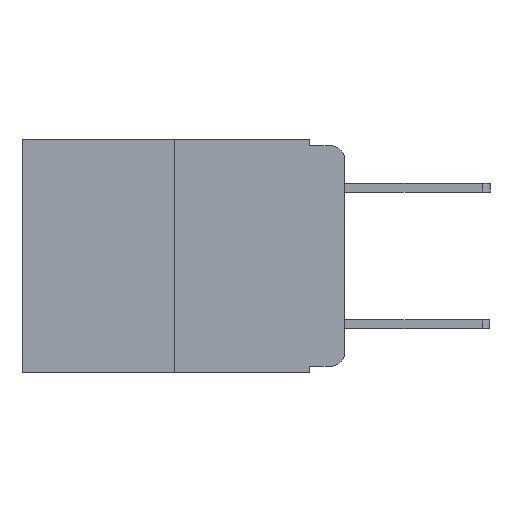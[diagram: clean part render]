
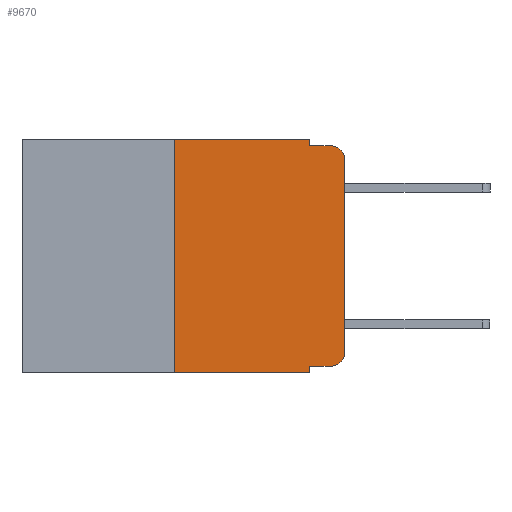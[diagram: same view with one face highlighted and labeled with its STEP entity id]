
A CAD part, left-side view. The second image highlights one B-rep face of the part: STEP entity #9670.
In plain terms, the highlighted planar face has unit normal (-1, 0, 0).
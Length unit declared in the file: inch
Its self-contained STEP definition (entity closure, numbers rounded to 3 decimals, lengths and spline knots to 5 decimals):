
#8 = LINE ( 'NONE', #18733, #17541 ) ;
#516 = DIRECTION ( 'NONE',  ( -1., 0., 0. ) ) ;
#666 = EDGE_CURVE ( 'NONE', #3687, #9447, #8, .T. ) ;
#792 = CARTESIAN_POINT ( 'NONE',  ( 0., 0.051, 0. ) ) ;
#981 = ORIENTED_EDGE ( 'NONE', *, *, #666, .T. ) ;
#1215 = ORIENTED_EDGE ( 'NONE', *, *, #8685, .F. ) ;
#2096 = VERTEX_POINT ( 'NONE', #7950 ) ;
#2182 = CARTESIAN_POINT ( 'NONE',  ( 0., 0.25, 0. ) ) ;
#2945 = EDGE_LOOP ( 'NONE', ( #5885, #19384, #20901, #8991, #1215, #12058, #11297, #17160, #981, #9784 ) ) ;
#3026 = LINE ( 'NONE', #5158, #6870 ) ;
#3411 = VERTEX_POINT ( 'NONE', #9431 ) ;
#3503 = LINE ( 'NONE', #6610, #16013 ) ;
#3687 = VERTEX_POINT ( 'NONE', #15047 ) ;
#3809 = CARTESIAN_POINT ( 'NONE',  ( 0., 0., 0. ) ) ;
#3881 = DIRECTION ( 'NONE',  ( 0., 0., 1. ) ) ;
#3888 = LINE ( 'NONE', #5105, #7714 ) ;
#3938 = VECTOR ( 'NONE', #11403, 39.37008 ) ;
#4030 = LINE ( 'NONE', #3809, #20818 ) ;
#4268 = EDGE_CURVE ( 'NONE', #18880, #7314, #3026, .T. ) ;
#4490 = DIRECTION ( 'NONE',  ( 1., 0., 0. ) ) ;
#4887 = CARTESIAN_POINT ( 'NONE',  ( 0., 0.25, 0. ) ) ;
#5105 = CARTESIAN_POINT ( 'NONE',  ( 0., 0.473, -0.343 ) ) ;
#5158 = CARTESIAN_POINT ( 'NONE',  ( 0., 0.051, 0. ) ) ;
#5649 = DIRECTION ( 'NONE',  ( -1., 0., 0. ) ) ;
#5885 = ORIENTED_EDGE ( 'NONE', *, *, #7518, .T. ) ;
#6610 = CARTESIAN_POINT ( 'NONE',  ( 0., 0.473, 0. ) ) ;
#6811 = DIRECTION ( 'NONE',  ( 0., 0., -1. ) ) ;
#6870 = VECTOR ( 'NONE', #6811, 39.37008 ) ;
#6994 = CIRCLE ( 'NONE', #13100, 0.02 ) ;
#7314 = VERTEX_POINT ( 'NONE', #18001 ) ;
#7518 = EDGE_CURVE ( 'NONE', #12707, #2096, #4030, .T. ) ;
#7714 = VECTOR ( 'NONE', #10047, 39.37008 ) ;
#7950 = CARTESIAN_POINT ( 'NONE',  ( 0., 0., -0.03 ) ) ;
#8685 = EDGE_CURVE ( 'NONE', #11737, #18880, #3503, .T. ) ;
#8953 = VECTOR ( 'NONE', #20118, 39.37008 ) ;
#8991 = ORIENTED_EDGE ( 'NONE', *, *, #4268, .F. ) ;
#9375 = CARTESIAN_POINT ( 'NONE',  ( 0., 0.473, 0. ) ) ;
#9431 = CARTESIAN_POINT ( 'NONE',  ( 0., 0.25, -0.343 ) ) ;
#9438 = LINE ( 'NONE', #792, #20835 ) ;
#9447 = VERTEX_POINT ( 'NONE', #15290 ) ;
#9456 = CARTESIAN_POINT ( 'NONE',  ( 0., 0.02, -0.01 ) ) ;
#9472 = LINE ( 'NONE', #18502, #8953 ) ;
#9670 = ADVANCED_FACE ( 'NONE', ( #18740 ), #20707, .F. ) ;
#9784 = ORIENTED_EDGE ( 'NONE', *, *, #10761, .T. ) ;
#10047 = DIRECTION ( 'NONE',  ( 0., -1., 0. ) ) ;
#10443 = CARTESIAN_POINT ( 'NONE',  ( 0., 0.02, -0.03 ) ) ;
#10444 = EDGE_CURVE ( 'NONE', #3411, #11737, #16956, .T. ) ;
#10761 = EDGE_CURVE ( 'NONE', #9447, #12707, #6994, .T. ) ;
#11297 = ORIENTED_EDGE ( 'NONE', *, *, #21209, .T. ) ;
#11338 = EDGE_CURVE ( 'NONE', #2096, #17224, #17426, .T. ) ;
#11403 = DIRECTION ( 'NONE',  ( 0., 0., 1. ) ) ;
#11737 = VERTEX_POINT ( 'NONE', #2182 ) ;
#12058 = ORIENTED_EDGE ( 'NONE', *, *, #10444, .F. ) ;
#12079 = DIRECTION ( 'NONE',  ( 0., 0., -1. ) ) ;
#12707 = VERTEX_POINT ( 'NONE', #18022 ) ;
#12909 = EDGE_CURVE ( 'NONE', #7314, #17224, #9472, .T. ) ;
#13100 = AXIS2_PLACEMENT_3D ( 'NONE', #15450, #5649, #17083 ) ;
#13389 = AXIS2_PLACEMENT_3D ( 'NONE', #10443, #516, #12079 ) ;
#14003 = CARTESIAN_POINT ( 'NONE',  ( 0., 0.051, -0.343 ) ) ;
#15047 = CARTESIAN_POINT ( 'NONE',  ( 0., 0.051, -0.333 ) ) ;
#15290 = CARTESIAN_POINT ( 'NONE',  ( 0., 0.02, -0.333 ) ) ;
#15450 = CARTESIAN_POINT ( 'NONE',  ( 0., 0.02, -0.313 ) ) ;
#15498 = DIRECTION ( 'NONE',  ( 0., -1., 0. ) ) ;
#15624 = DIRECTION ( 'NONE',  ( 0., 0., -1. ) ) ;
#15912 = DIRECTION ( 'NONE',  ( 0., 0., -1. ) ) ;
#16013 = VECTOR ( 'NONE', #18003, 39.37008 ) ;
#16411 = VERTEX_POINT ( 'NONE', #14003 ) ;
#16956 = LINE ( 'NONE', #4887, #3938 ) ;
#17083 = DIRECTION ( 'NONE',  ( 0., 0., -1. ) ) ;
#17160 = ORIENTED_EDGE ( 'NONE', *, *, #19131, .F. ) ;
#17224 = VERTEX_POINT ( 'NONE', #9456 ) ;
#17426 = CIRCLE ( 'NONE', #13389, 0.02 ) ;
#17541 = VECTOR ( 'NONE', #15498, 39.37008 ) ;
#18001 = CARTESIAN_POINT ( 'NONE',  ( 0., 0.051, -0.01 ) ) ;
#18003 = DIRECTION ( 'NONE',  ( 0., -1., 0. ) ) ;
#18022 = CARTESIAN_POINT ( 'NONE',  ( 0., 0., -0.313 ) ) ;
#18502 = CARTESIAN_POINT ( 'NONE',  ( 0., 0.051, -0.01 ) ) ;
#18733 = CARTESIAN_POINT ( 'NONE',  ( 0., 0.051, -0.333 ) ) ;
#18740 = FACE_OUTER_BOUND ( 'NONE', #2945, .T. ) ;
#18880 = VERTEX_POINT ( 'NONE', #19781 ) ;
#19131 = EDGE_CURVE ( 'NONE', #3687, #16411, #9438, .T. ) ;
#19384 = ORIENTED_EDGE ( 'NONE', *, *, #11338, .T. ) ;
#19781 = CARTESIAN_POINT ( 'NONE',  ( 0., 0.051, 0. ) ) ;
#20106 = AXIS2_PLACEMENT_3D ( 'NONE', #9375, #4490, #15912 ) ;
#20118 = DIRECTION ( 'NONE',  ( 0., -1., 0. ) ) ;
#20707 = PLANE ( 'NONE',  #20106 ) ;
#20818 = VECTOR ( 'NONE', #3881, 39.37008 ) ;
#20835 = VECTOR ( 'NONE', #15624, 39.37008 ) ;
#20901 = ORIENTED_EDGE ( 'NONE', *, *, #12909, .F. ) ;
#21209 = EDGE_CURVE ( 'NONE', #3411, #16411, #3888, .T. ) ;
